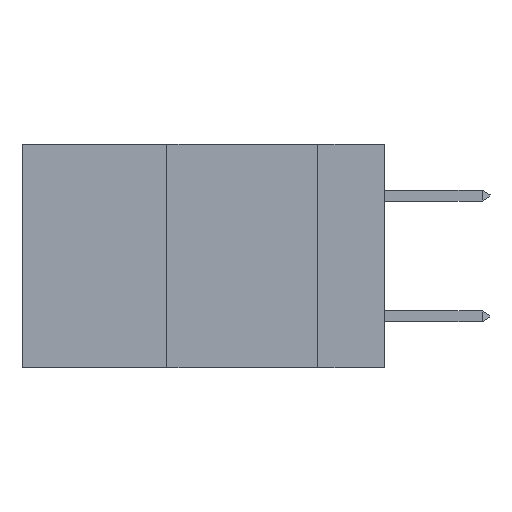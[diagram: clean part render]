
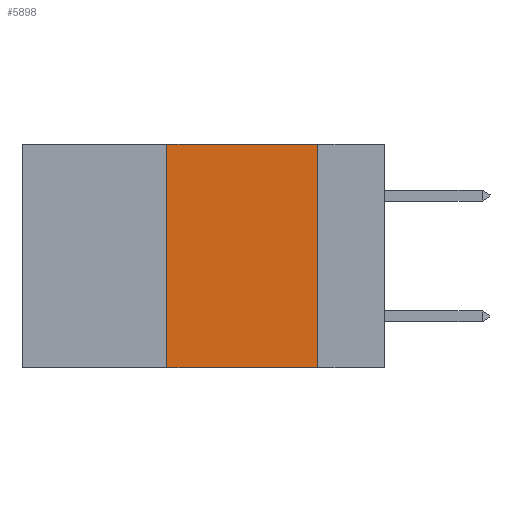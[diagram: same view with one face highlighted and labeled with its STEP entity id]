
A CAD part, left-side view. The second image highlights one B-rep face of the part: STEP entity #5898.
In plain terms, the highlighted planar face has unit normal (-1, 0, 0).
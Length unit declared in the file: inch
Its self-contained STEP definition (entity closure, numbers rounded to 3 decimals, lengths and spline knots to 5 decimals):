
#13 = LINE ( 'NONE', #16992, #5497 ) ;
#3242 = VERTEX_POINT ( 'NONE', #26632 ) ;
#3810 = CARTESIAN_POINT ( 'NONE',  ( 0., 0.6, 0. ) ) ;
#4972 = CARTESIAN_POINT ( 'NONE',  ( 0., 0.6, 0. ) ) ;
#5257 = DIRECTION ( 'NONE',  ( 0., 0., 1. ) ) ;
#5497 = VECTOR ( 'NONE', #5257, 39.37008 ) ;
#5898 = ADVANCED_FACE ( 'NONE', ( #17673 ), #6136, .F. ) ;
#6136 = PLANE ( 'NONE',  #24260 ) ;
#8505 = DIRECTION ( 'NONE',  ( 0., 0., -1. ) ) ;
#8525 = VECTOR ( 'NONE', #16694, 39.37008 ) ;
#9793 = ORIENTED_EDGE ( 'NONE', *, *, #20171, .F. ) ;
#10178 = EDGE_LOOP ( 'NONE', ( #13079, #20881, #9793, #23851 ) ) ;
#10454 = DIRECTION ( 'NONE',  ( 0., -1., 0. ) ) ;
#10590 = CARTESIAN_POINT ( 'NONE',  ( 0., 0.11, 0. ) ) ;
#13079 = ORIENTED_EDGE ( 'NONE', *, *, #26520, .F. ) ;
#13420 = VECTOR ( 'NONE', #24765, 39.37008 ) ;
#13805 = EDGE_CURVE ( 'NONE', #14974, #17189, #27588, .T. ) ;
#14758 = LINE ( 'NONE', #4972, #8525 ) ;
#14974 = VERTEX_POINT ( 'NONE', #30257 ) ;
#16415 = CARTESIAN_POINT ( 'NONE',  ( 0., 0.36, 0. ) ) ;
#16694 = DIRECTION ( 'NONE',  ( 0., -1., 0. ) ) ;
#16992 = CARTESIAN_POINT ( 'NONE',  ( 0., 0.36, 0. ) ) ;
#17189 = VERTEX_POINT ( 'NONE', #19284 ) ;
#17673 = FACE_OUTER_BOUND ( 'NONE', #10178, .T. ) ;
#18045 = EDGE_CURVE ( 'NONE', #29143, #3242, #14758, .T. ) ;
#19284 = CARTESIAN_POINT ( 'NONE',  ( 0., 0.11, -0.37 ) ) ;
#20171 = EDGE_CURVE ( 'NONE', #14974, #29143, #13, .T. ) ;
#20881 = ORIENTED_EDGE ( 'NONE', *, *, #18045, .F. ) ;
#22034 = VECTOR ( 'NONE', #10454, 39.37008 ) ;
#22633 = DIRECTION ( 'NONE',  ( 1., 0., 0. ) ) ;
#23851 = ORIENTED_EDGE ( 'NONE', *, *, #13805, .T. ) ;
#24260 = AXIS2_PLACEMENT_3D ( 'NONE', #3810, #22633, #8505 ) ;
#24765 = DIRECTION ( 'NONE',  ( 0., 0., -1. ) ) ;
#26038 = LINE ( 'NONE', #10590, #13420 ) ;
#26520 = EDGE_CURVE ( 'NONE', #3242, #17189, #26038, .T. ) ;
#26632 = CARTESIAN_POINT ( 'NONE',  ( 0., 0.11, 0. ) ) ;
#27588 = LINE ( 'NONE', #29474, #22034 ) ;
#29143 = VERTEX_POINT ( 'NONE', #16415 ) ;
#29474 = CARTESIAN_POINT ( 'NONE',  ( 0., 0.6, -0.37 ) ) ;
#30257 = CARTESIAN_POINT ( 'NONE',  ( 0., 0.36, -0.37 ) ) ;
